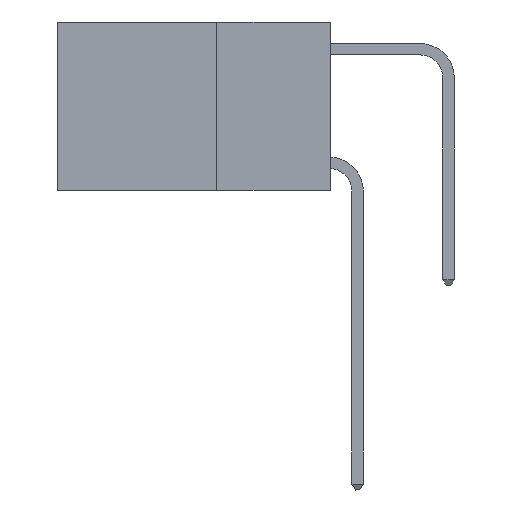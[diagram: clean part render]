
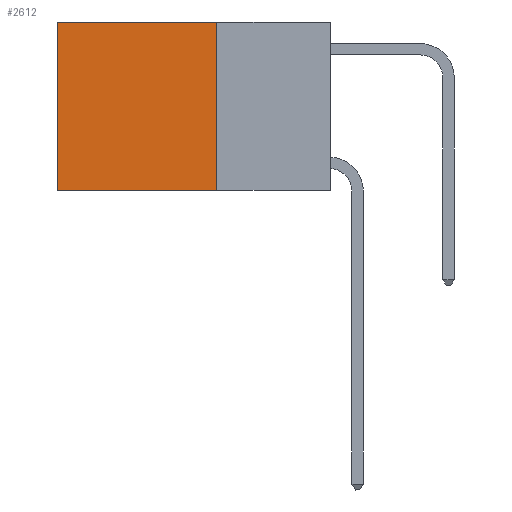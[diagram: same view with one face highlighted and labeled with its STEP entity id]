
A CAD part, left-side view. The second image highlights one B-rep face of the part: STEP entity #2612.
In plain terms, the highlighted planar face has unit normal (-1, 0, 0).
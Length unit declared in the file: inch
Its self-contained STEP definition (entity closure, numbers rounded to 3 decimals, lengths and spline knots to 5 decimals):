
#134 = CARTESIAN_POINT ( 'NONE',  ( 0.2625, 0.25, 0. ) ) ;
#1190 = DIRECTION ( 'NONE',  ( 0., 1., 0. ) ) ;
#1393 = CARTESIAN_POINT ( 'NONE',  ( 0.2625, 0.25, 0. ) ) ;
#1532 = VECTOR ( 'NONE', #1190, 39.37008 ) ;
#2612 = ADVANCED_FACE ( 'NONE', ( #29737 ), #25497, .F. ) ;
#3234 = DIRECTION ( 'NONE',  ( 0., 1., 0. ) ) ;
#5176 = CARTESIAN_POINT ( 'NONE',  ( 0.2625, 0.25, 0. ) ) ;
#6906 = CARTESIAN_POINT ( 'NONE',  ( 0.2625, 0.6, 0. ) ) ;
#8566 = CARTESIAN_POINT ( 'NONE',  ( 0.2625, 0.25, 0. ) ) ;
#9541 = DIRECTION ( 'NONE',  ( 1., 0., 0. ) ) ;
#9615 = DIRECTION ( 'NONE',  ( 0., 0., -1. ) ) ;
#9786 = CARTESIAN_POINT ( 'NONE',  ( 0.2625, 0.6, 0. ) ) ;
#9861 = LINE ( 'NONE', #134, #31048 ) ;
#10552 = EDGE_CURVE ( 'NONE', #22451, #25583, #26142, .T. ) ;
#10583 = VECTOR ( 'NONE', #9615, 39.37008 ) ;
#10854 = DIRECTION ( 'NONE',  ( 0., 0., -1. ) ) ;
#11037 = VERTEX_POINT ( 'NONE', #23789 ) ;
#12718 = EDGE_CURVE ( 'NONE', #25583, #11037, #32604, .T. ) ;
#13874 = ORIENTED_EDGE ( 'NONE', *, *, #22084, .F. ) ;
#17155 = CARTESIAN_POINT ( 'NONE',  ( 0.2625, 0.25, -0.37 ) ) ;
#18266 = VECTOR ( 'NONE', #3234, 39.37008 ) ;
#19203 = AXIS2_PLACEMENT_3D ( 'NONE', #1393, #9541, #28131 ) ;
#20345 = ORIENTED_EDGE ( 'NONE', *, *, #10552, .T. ) ;
#22084 = EDGE_CURVE ( 'NONE', #32365, #11037, #29934, .T. ) ;
#22216 = EDGE_LOOP ( 'NONE', ( #27378, #13874, #28715, #20345 ) ) ;
#22451 = VERTEX_POINT ( 'NONE', #5176 ) ;
#23789 = CARTESIAN_POINT ( 'NONE',  ( 0.2625, 0.6, -0.37 ) ) ;
#25497 = PLANE ( 'NONE',  #19203 ) ;
#25583 = VERTEX_POINT ( 'NONE', #9786 ) ;
#25625 = CARTESIAN_POINT ( 'NONE',  ( 0.2625, 0.25, -0.37 ) ) ;
#26142 = LINE ( 'NONE', #8566, #18266 ) ;
#27378 = ORIENTED_EDGE ( 'NONE', *, *, #12718, .T. ) ;
#28131 = DIRECTION ( 'NONE',  ( 0., 0., -1. ) ) ;
#28715 = ORIENTED_EDGE ( 'NONE', *, *, #31363, .F. ) ;
#29737 = FACE_OUTER_BOUND ( 'NONE', #22216, .T. ) ;
#29934 = LINE ( 'NONE', #17155, #1532 ) ;
#31048 = VECTOR ( 'NONE', #10854, 39.37008 ) ;
#31363 = EDGE_CURVE ( 'NONE', #22451, #32365, #9861, .T. ) ;
#32365 = VERTEX_POINT ( 'NONE', #25625 ) ;
#32604 = LINE ( 'NONE', #6906, #10583 ) ;
